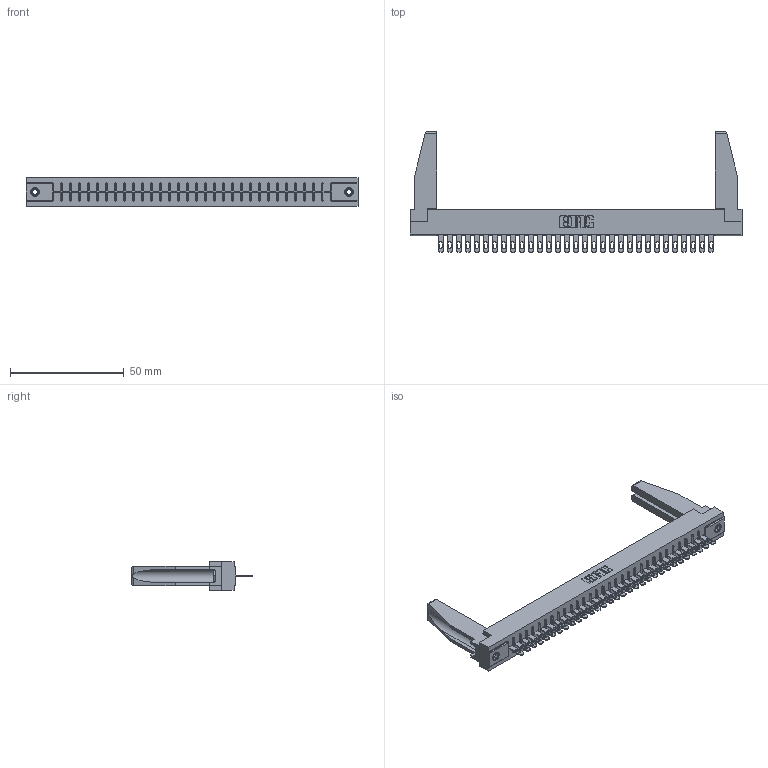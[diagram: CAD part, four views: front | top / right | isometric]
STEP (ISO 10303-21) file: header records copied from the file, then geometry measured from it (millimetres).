
FILE_DESCRIPTION (( 'STEP AP203' ), '1' );
FILE_NAME ('356-031-400-178.STEP', '2020-09-23T20:47:39', ( '' ), ( '' ), 'SwSTEP 2.0', 'SolidWorks 2020', '' );
FILE_SCHEMA (( 'CONFIG_CONTROL_DESIGN' ));
Length unit declared in the file: inch
Products named in the file (5): 307-220-078; 306 Part_.156 Dia; 356-031-400-178; 306-290-001_100; 345-250-001_345-250-001-102
Assembly tree (36 placements, depth 2):
  356-031-400-178
    306 Part_.156 Dia
    306-290-001_100  x31
    345-250-001_345-250-001-102  x2
    307-220-078  x2
Bounding box: 145.85 x 52.91 x 12.7 mm (x, y, z)
Volume: 20119.1 mm3; surface area: 20813.3 mm2
Topology: 36 solids, 36 shells, 2602 faces, 7311 edges, 4698 vertices
Faces by surface type: plane 1702, cylinder 760, sphere 124, cone 12, torus 4
Entity records: 32937 total; most frequent: CARTESIAN_POINT 5530, ORIENTED_EDGE 5440, DIRECTION 5406, EDGE_CURVE 2720, LINE 2122, VECTOR 2122, VERTEX_POINT 1724, AXIS2_PLACEMENT_3D 1642
